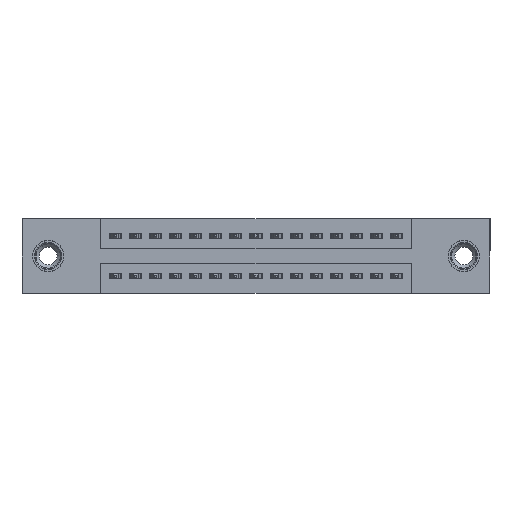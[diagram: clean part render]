
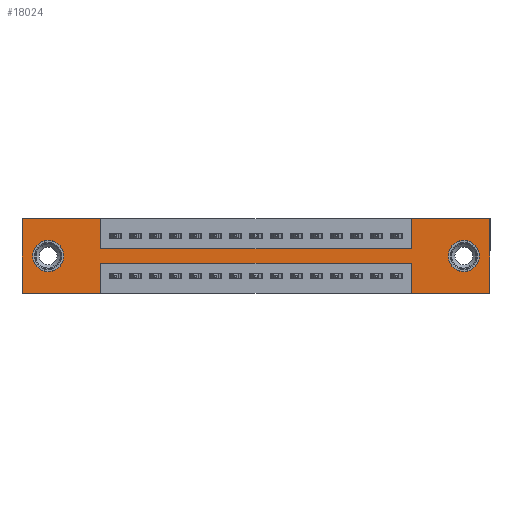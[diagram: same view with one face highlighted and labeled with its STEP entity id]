
A CAD part, front view. The second image highlights one B-rep face of the part: STEP entity #18024.
In plain terms, the highlighted planar face has unit normal (0, -1, 0).
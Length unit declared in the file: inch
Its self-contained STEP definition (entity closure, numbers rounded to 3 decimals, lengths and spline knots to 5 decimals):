
#95 = EDGE_CURVE ( 'NONE', #10896, #11611, #17291, .T. ) ;
#386 = VECTOR ( 'NONE', #6343, 39.37008 ) ;
#511 = CARTESIAN_POINT ( 'NONE',  ( 0.3925, 0., -0.15 ) ) ;
#548 = CARTESIAN_POINT ( 'NONE',  ( 0., 0., -0.37 ) ) ;
#597 = PLANE ( 'NONE',  #8467 ) ;
#616 = VECTOR ( 'NONE', #2809, 39.37008 ) ;
#659 = AXIS2_PLACEMENT_3D ( 'NONE', #12685, #3575, #14270 ) ;
#763 = ORIENTED_EDGE ( 'NONE', *, *, #14628, .T. ) ;
#870 = ORIENTED_EDGE ( 'NONE', *, *, #8961, .F. ) ;
#873 = EDGE_CURVE ( 'NONE', #12317, #12097, #8875, .T. ) ;
#941 = ORIENTED_EDGE ( 'NONE', *, *, #7421, .T. ) ;
#1272 = CARTESIAN_POINT ( 'NONE',  ( 1.9425, 0., 0. ) ) ;
#1361 = VERTEX_POINT ( 'NONE', #1272 ) ;
#1556 = ORIENTED_EDGE ( 'NONE', *, *, #95, .F. ) ;
#1581 = VERTEX_POINT ( 'NONE', #3330 ) ;
#1816 = VECTOR ( 'NONE', #4293, 39.37008 ) ;
#1974 = VERTEX_POINT ( 'NONE', #15383 ) ;
#2137 = CARTESIAN_POINT ( 'NONE',  ( 0., 0., 0. ) ) ;
#2159 = VECTOR ( 'NONE', #17485, 39.37008 ) ;
#2183 = CARTESIAN_POINT ( 'NONE',  ( 0., 0., 0. ) ) ;
#2253 = VERTEX_POINT ( 'NONE', #11572 ) ;
#2364 = DIRECTION ( 'NONE',  ( 0., 0., -1. ) ) ;
#2581 = FACE_OUTER_BOUND ( 'NONE', #16963, .T. ) ;
#2598 = ORIENTED_EDGE ( 'NONE', *, *, #15641, .F. ) ;
#2621 = EDGE_CURVE ( 'NONE', #13540, #12317, #7382, .T. ) ;
#2809 = DIRECTION ( 'NONE',  ( 0., 0., 1. ) ) ;
#3036 = DIRECTION ( 'NONE',  ( 0., 1., 0. ) ) ;
#3213 = VERTEX_POINT ( 'NONE', #7188 ) ;
#3264 = VECTOR ( 'NONE', #7946, 39.37008 ) ;
#3297 = CARTESIAN_POINT ( 'NONE',  ( 2.205, 0., -0.263 ) ) ;
#3330 = CARTESIAN_POINT ( 'NONE',  ( 0.3925, 0., -0.15 ) ) ;
#3575 = DIRECTION ( 'NONE',  ( 0., 1., 0. ) ) ;
#3689 = CARTESIAN_POINT ( 'NONE',  ( 0.3925, 0., -0.22 ) ) ;
#4272 = CARTESIAN_POINT ( 'NONE',  ( 0., 0., 0. ) ) ;
#4293 = DIRECTION ( 'NONE',  ( 1., 0., 0. ) ) ;
#4319 = DIRECTION ( 'NONE',  ( 0., 0., 1. ) ) ;
#4731 = AXIS2_PLACEMENT_3D ( 'NONE', #18222, #9071, #19755 ) ;
#5085 = DIRECTION ( 'NONE',  ( 0., 1., 0. ) ) ;
#5306 = FACE_BOUND ( 'NONE', #7783, .T. ) ;
#5507 = CIRCLE ( 'NONE', #12106, 0.078 ) ;
#5584 = EDGE_CURVE ( 'NONE', #12097, #2253, #6375, .T. ) ;
#5944 = DIRECTION ( 'NONE',  ( 0., 0., -1. ) ) ;
#6062 = VERTEX_POINT ( 'NONE', #548 ) ;
#6140 = ORIENTED_EDGE ( 'NONE', *, *, #2621, .F. ) ;
#6272 = LINE ( 'NONE', #9374, #13875 ) ;
#6343 = DIRECTION ( 'NONE',  ( -1., 0., 0. ) ) ;
#6362 = LINE ( 'NONE', #3689, #2159 ) ;
#6375 = LINE ( 'NONE', #11860, #18062 ) ;
#6454 = VERTEX_POINT ( 'NONE', #11164 ) ;
#6620 = ORIENTED_EDGE ( 'NONE', *, *, #13158, .F. ) ;
#6663 = CARTESIAN_POINT ( 'NONE',  ( 0., 0., -0.37 ) ) ;
#6697 = ORIENTED_EDGE ( 'NONE', *, *, #18364, .F. ) ;
#6918 = EDGE_CURVE ( 'NONE', #9373, #17773, #7259, .T. ) ;
#6969 = ORIENTED_EDGE ( 'NONE', *, *, #9399, .F. ) ;
#7063 = AXIS2_PLACEMENT_3D ( 'NONE', #12177, #3036, #13765 ) ;
#7188 = CARTESIAN_POINT ( 'NONE',  ( 0.13, 0., -0.107 ) ) ;
#7259 = CIRCLE ( 'NONE', #4731, 0.078 ) ;
#7382 = LINE ( 'NONE', #20006, #3264 ) ;
#7421 = EDGE_CURVE ( 'NONE', #3213, #12944, #10279, .T. ) ;
#7594 = VECTOR ( 'NONE', #13363, 39.37008 ) ;
#7615 = VECTOR ( 'NONE', #10542, 39.37008 ) ;
#7783 = EDGE_LOOP ( 'NONE', ( #941, #9011 ) ) ;
#7855 = DIRECTION ( 'NONE',  ( 0., 0., -1. ) ) ;
#7946 = DIRECTION ( 'NONE',  ( 0., 0., -1. ) ) ;
#8084 = LINE ( 'NONE', #11803, #7594 ) ;
#8467 = AXIS2_PLACEMENT_3D ( 'NONE', #17726, #11557, #2364 ) ;
#8610 = LINE ( 'NONE', #11954, #616 ) ;
#8875 = LINE ( 'NONE', #16620, #386 ) ;
#8961 = EDGE_CURVE ( 'NONE', #6454, #10397, #16502, .T. ) ;
#9011 = ORIENTED_EDGE ( 'NONE', *, *, #10238, .T. ) ;
#9071 = DIRECTION ( 'NONE',  ( 0., 1., 0. ) ) ;
#9373 = VERTEX_POINT ( 'NONE', #9824 ) ;
#9374 = CARTESIAN_POINT ( 'NONE',  ( 0.3925, 0., 0. ) ) ;
#9399 = EDGE_CURVE ( 'NONE', #6062, #10896, #16009, .T. ) ;
#9765 = CARTESIAN_POINT ( 'NONE',  ( 2.335, 0., 0. ) ) ;
#9824 = CARTESIAN_POINT ( 'NONE',  ( 2.205, 0., -0.107 ) ) ;
#10145 = EDGE_LOOP ( 'NONE', ( #15868, #763 ) ) ;
#10183 = CARTESIAN_POINT ( 'NONE',  ( 0.3925, 0., -0.37 ) ) ;
#10238 = EDGE_CURVE ( 'NONE', #12944, #3213, #5507, .T. ) ;
#10279 = CIRCLE ( 'NONE', #7063, 0.078 ) ;
#10294 = CARTESIAN_POINT ( 'NONE',  ( 1.9425, 0., -0.37 ) ) ;
#10397 = VERTEX_POINT ( 'NONE', #10183 ) ;
#10438 = CARTESIAN_POINT ( 'NONE',  ( 0.3925, 0., 0. ) ) ;
#10542 = DIRECTION ( 'NONE',  ( 1., 0., 0. ) ) ;
#10766 = ORIENTED_EDGE ( 'NONE', *, *, #12131, .F. ) ;
#10896 = VERTEX_POINT ( 'NONE', #2137 ) ;
#10941 = ORIENTED_EDGE ( 'NONE', *, *, #13484, .F. ) ;
#11137 = ORIENTED_EDGE ( 'NONE', *, *, #12667, .F. ) ;
#11164 = CARTESIAN_POINT ( 'NONE',  ( 0.3925, 0., -0.22 ) ) ;
#11389 = DIRECTION ( 'NONE',  ( 0., 0., 1. ) ) ;
#11557 = DIRECTION ( 'NONE',  ( 0., -1., 0. ) ) ;
#11572 = CARTESIAN_POINT ( 'NONE',  ( 1.9425, 0., -0.22 ) ) ;
#11611 = VERTEX_POINT ( 'NONE', #10438 ) ;
#11614 = LINE ( 'NONE', #511, #7615 ) ;
#11803 = CARTESIAN_POINT ( 'NONE',  ( 0., 0., 0. ) ) ;
#11860 = CARTESIAN_POINT ( 'NONE',  ( 1.9425, 0., -0.37 ) ) ;
#11954 = CARTESIAN_POINT ( 'NONE',  ( 1.9425, 0., 0. ) ) ;
#12097 = VERTEX_POINT ( 'NONE', #10294 ) ;
#12106 = AXIS2_PLACEMENT_3D ( 'NONE', #14220, #5085, #15776 ) ;
#12131 = EDGE_CURVE ( 'NONE', #1974, #1361, #8610, .T. ) ;
#12177 = CARTESIAN_POINT ( 'NONE',  ( 0.13, 0., -0.185 ) ) ;
#12317 = VERTEX_POINT ( 'NONE', #18415 ) ;
#12333 = VECTOR ( 'NONE', #11389, 39.37008 ) ;
#12372 = ORIENTED_EDGE ( 'NONE', *, *, #5584, .F. ) ;
#12667 = EDGE_CURVE ( 'NONE', #1581, #1974, #11614, .T. ) ;
#12685 = CARTESIAN_POINT ( 'NONE',  ( 2.205, 0., -0.185 ) ) ;
#12944 = VERTEX_POINT ( 'NONE', #17307 ) ;
#13158 = EDGE_CURVE ( 'NONE', #1361, #13540, #8084, .T. ) ;
#13363 = DIRECTION ( 'NONE',  ( 1., 0., 0. ) ) ;
#13373 = FACE_BOUND ( 'NONE', #10145, .T. ) ;
#13484 = EDGE_CURVE ( 'NONE', #10397, #6062, #14021, .T. ) ;
#13540 = VERTEX_POINT ( 'NONE', #9765 ) ;
#13765 = DIRECTION ( 'NONE',  ( 0., 0., 1. ) ) ;
#13875 = VECTOR ( 'NONE', #7855, 39.37008 ) ;
#14021 = LINE ( 'NONE', #6663, #18101 ) ;
#14220 = CARTESIAN_POINT ( 'NONE',  ( 0.13, 0., -0.185 ) ) ;
#14270 = DIRECTION ( 'NONE',  ( 0., 0., -1. ) ) ;
#14628 = EDGE_CURVE ( 'NONE', #17773, #9373, #19722, .T. ) ;
#14990 = CARTESIAN_POINT ( 'NONE',  ( 0.3925, 0., -0.37 ) ) ;
#15383 = CARTESIAN_POINT ( 'NONE',  ( 1.9425, 0., -0.15 ) ) ;
#15641 = EDGE_CURVE ( 'NONE', #2253, #6454, #6362, .T. ) ;
#15776 = DIRECTION ( 'NONE',  ( 0., 0., 1. ) ) ;
#15868 = ORIENTED_EDGE ( 'NONE', *, *, #6918, .T. ) ;
#16009 = LINE ( 'NONE', #2183, #12333 ) ;
#16331 = ORIENTED_EDGE ( 'NONE', *, *, #873, .F. ) ;
#16502 = LINE ( 'NONE', #14990, #20063 ) ;
#16620 = CARTESIAN_POINT ( 'NONE',  ( 0., 0., -0.37 ) ) ;
#16963 = EDGE_LOOP ( 'NONE', ( #870, #2598, #12372, #16331, #6140, #6620, #10766, #11137, #6697, #1556, #6969, #10941 ) ) ;
#17291 = LINE ( 'NONE', #4272, #1816 ) ;
#17307 = CARTESIAN_POINT ( 'NONE',  ( 0.13, 0., -0.263 ) ) ;
#17353 = DIRECTION ( 'NONE',  ( -1., 0., 0. ) ) ;
#17485 = DIRECTION ( 'NONE',  ( -1., 0., 0. ) ) ;
#17726 = CARTESIAN_POINT ( 'NONE',  ( 0., 0., -0.37 ) ) ;
#17773 = VERTEX_POINT ( 'NONE', #3297 ) ;
#18024 = ADVANCED_FACE ( 'NONE', ( #13373, #5306, #2581 ), #597, .T. ) ;
#18062 = VECTOR ( 'NONE', #4319, 39.37008 ) ;
#18101 = VECTOR ( 'NONE', #17353, 39.37008 ) ;
#18222 = CARTESIAN_POINT ( 'NONE',  ( 2.205, 0., -0.185 ) ) ;
#18364 = EDGE_CURVE ( 'NONE', #11611, #1581, #6272, .T. ) ;
#18415 = CARTESIAN_POINT ( 'NONE',  ( 2.335, 0., -0.37 ) ) ;
#19722 = CIRCLE ( 'NONE', #659, 0.078 ) ;
#19755 = DIRECTION ( 'NONE',  ( 0., 0., -1. ) ) ;
#20006 = CARTESIAN_POINT ( 'NONE',  ( 2.335, 0., 0. ) ) ;
#20063 = VECTOR ( 'NONE', #5944, 39.37008 ) ;
